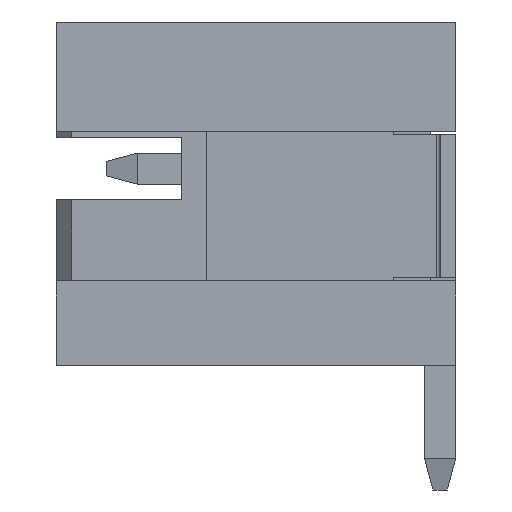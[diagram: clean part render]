
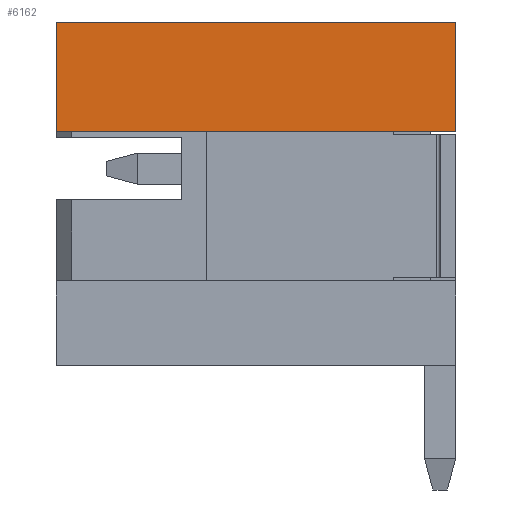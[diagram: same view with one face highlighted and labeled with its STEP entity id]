
A CAD part, left-side view. The second image highlights one B-rep face of the part: STEP entity #6162.
In plain terms, the highlighted planar face has unit normal (-1, 0, 0).
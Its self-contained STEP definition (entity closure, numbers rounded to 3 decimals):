
#69 = CARTESIAN_POINT ( 'NONE',  ( -3., 0., 2.35 ) ) ;
#208 = CARTESIAN_POINT ( 'NONE',  ( -3., 0., 0. ) ) ;
#264 = AXIS2_PLACEMENT_3D ( 'NONE', #208, #808, #7689 ) ;
#362 = ORIENTED_EDGE ( 'NONE', *, *, #3778, .F. ) ;
#750 = CARTESIAN_POINT ( 'NONE',  ( -3., 6.4, 2.35 ) ) ;
#808 = DIRECTION ( 'NONE',  ( 1., 0., 0. ) ) ;
#1010 = CARTESIAN_POINT ( 'NONE',  ( -3., 0., 2.35 ) ) ;
#1463 = DIRECTION ( 'NONE',  ( 0., 1., 0. ) ) ;
#1665 = EDGE_LOOP ( 'NONE', ( #4476, #2132, #5048, #362 ) ) ;
#2132 = ORIENTED_EDGE ( 'NONE', *, *, #4763, .F. ) ;
#2350 = VERTEX_POINT ( 'NONE', #6244 ) ;
#2759 = LINE ( 'NONE', #69, #3922 ) ;
#2785 = DIRECTION ( 'NONE',  ( 0., 0., 1. ) ) ;
#2892 = PLANE ( 'NONE',  #264 ) ;
#2896 = VECTOR ( 'NONE', #1463, 1000. ) ;
#3000 = LINE ( 'NONE', #5524, #2896 ) ;
#3308 = DIRECTION ( 'NONE',  ( 0., -1., 0. ) ) ;
#3756 = LINE ( 'NONE', #750, #5791 ) ;
#3778 = EDGE_CURVE ( 'NONE', #5759, #6459, #4417, .T. ) ;
#3922 = VECTOR ( 'NONE', #8134, 1000. ) ;
#4037 = FACE_OUTER_BOUND ( 'NONE', #1665, .T. ) ;
#4417 = LINE ( 'NONE', #6001, #5703 ) ;
#4476 = ORIENTED_EDGE ( 'NONE', *, *, #8410, .F. ) ;
#4763 = EDGE_CURVE ( 'NONE', #7638, #2350, #3000, .T. ) ;
#5048 = ORIENTED_EDGE ( 'NONE', *, *, #6076, .F. ) ;
#5524 = CARTESIAN_POINT ( 'NONE',  ( -3., 0., 0.6 ) ) ;
#5703 = VECTOR ( 'NONE', #3308, 1000. ) ;
#5759 = VERTEX_POINT ( 'NONE', #8495 ) ;
#5791 = VECTOR ( 'NONE', #2785, 1000. ) ;
#6001 = CARTESIAN_POINT ( 'NONE',  ( -3., 6.4, 2.35 ) ) ;
#6074 = CARTESIAN_POINT ( 'NONE',  ( -3., 0., 0.6 ) ) ;
#6076 = EDGE_CURVE ( 'NONE', #6459, #7638, #2759, .T. ) ;
#6162 = ADVANCED_FACE ( 'NONE', ( #4037 ), #2892, .F. ) ;
#6244 = CARTESIAN_POINT ( 'NONE',  ( -3., 6.4, 0.6 ) ) ;
#6459 = VERTEX_POINT ( 'NONE', #1010 ) ;
#7638 = VERTEX_POINT ( 'NONE', #6074 ) ;
#7689 = DIRECTION ( 'NONE',  ( 0., 0., -1. ) ) ;
#8134 = DIRECTION ( 'NONE',  ( 0., 0., -1. ) ) ;
#8410 = EDGE_CURVE ( 'NONE', #2350, #5759, #3756, .T. ) ;
#8495 = CARTESIAN_POINT ( 'NONE',  ( -3., 6.4, 2.35 ) ) ;
